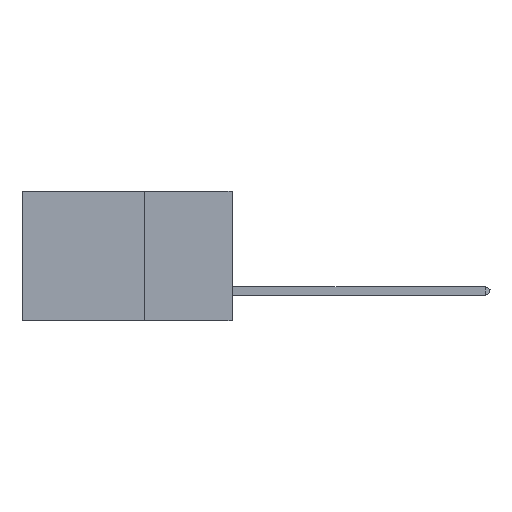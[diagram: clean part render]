
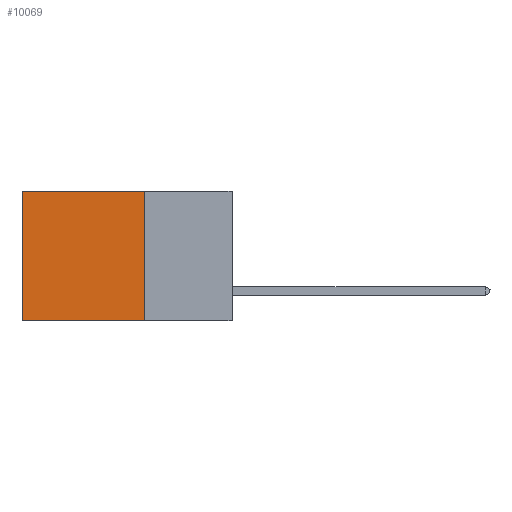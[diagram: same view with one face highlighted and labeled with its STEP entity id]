
A CAD part, left-side view. The second image highlights one B-rep face of the part: STEP entity #10069.
In plain terms, the highlighted planar face has unit normal (-1, 0, 0).
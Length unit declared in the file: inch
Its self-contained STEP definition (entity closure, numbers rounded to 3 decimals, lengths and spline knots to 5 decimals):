
#80 = VERTEX_POINT ( 'NONE', #22462 ) ;
#1959 = LINE ( 'NONE', #12753, #18884 ) ;
#3617 = ORIENTED_EDGE ( 'NONE', *, *, #5419, .T. ) ;
#4255 = CARTESIAN_POINT ( 'NONE',  ( 0.2875, 0.6, -0.37 ) ) ;
#4727 = EDGE_CURVE ( 'NONE', #80, #43732, #26885, .T. ) ;
#4766 = LINE ( 'NONE', #8727, #22227 ) ;
#5419 = EDGE_CURVE ( 'NONE', #16452, #80, #1959, .T. ) ;
#5517 = DIRECTION ( 'NONE',  ( 0., 0., -1. ) ) ;
#6976 = VECTOR ( 'NONE', #5517, 39.37008 ) ;
#8727 = CARTESIAN_POINT ( 'NONE',  ( 0.2875, 0.25, -0.37 ) ) ;
#9321 = DIRECTION ( 'NONE',  ( 0., 1., 0. ) ) ;
#9441 = DIRECTION ( 'NONE',  ( 0., 0., -1. ) ) ;
#10053 = PLANE ( 'NONE',  #28474 ) ;
#10069 = ADVANCED_FACE ( 'NONE', ( #41550 ), #10053, .F. ) ;
#10844 = ORIENTED_EDGE ( 'NONE', *, *, #43040, .F. ) ;
#12753 = CARTESIAN_POINT ( 'NONE',  ( 0.2875, 0.25, 0. ) ) ;
#13505 = DIRECTION ( 'NONE',  ( 0., 0., -1. ) ) ;
#13970 = ORIENTED_EDGE ( 'NONE', *, *, #28134, .F. ) ;
#14473 = CARTESIAN_POINT ( 'NONE',  ( 0.2875, 0.25, 0. ) ) ;
#16452 = VERTEX_POINT ( 'NONE', #23344 ) ;
#18884 = VECTOR ( 'NONE', #9321, 39.37008 ) ;
#19973 = CARTESIAN_POINT ( 'NONE',  ( 0.2875, 0.25, -0.37 ) ) ;
#20167 = CARTESIAN_POINT ( 'NONE',  ( 0.2875, 0.6, 0. ) ) ;
#22227 = VECTOR ( 'NONE', #30052, 39.37008 ) ;
#22462 = CARTESIAN_POINT ( 'NONE',  ( 0.2875, 0.6, 0. ) ) ;
#23344 = CARTESIAN_POINT ( 'NONE',  ( 0.2875, 0.25, 0. ) ) ;
#26885 = LINE ( 'NONE', #20167, #45029 ) ;
#27802 = CARTESIAN_POINT ( 'NONE',  ( 0.2875, 0.25, 0. ) ) ;
#28134 = EDGE_CURVE ( 'NONE', #16452, #32586, #46681, .T. ) ;
#28474 = AXIS2_PLACEMENT_3D ( 'NONE', #14473, #35374, #13505 ) ;
#30052 = DIRECTION ( 'NONE',  ( 0., 1., 0. ) ) ;
#32586 = VERTEX_POINT ( 'NONE', #19973 ) ;
#35374 = DIRECTION ( 'NONE',  ( 1., 0., 0. ) ) ;
#37618 = ORIENTED_EDGE ( 'NONE', *, *, #4727, .T. ) ;
#38547 = EDGE_LOOP ( 'NONE', ( #37618, #10844, #13970, #3617 ) ) ;
#41550 = FACE_OUTER_BOUND ( 'NONE', #38547, .T. ) ;
#43040 = EDGE_CURVE ( 'NONE', #32586, #43732, #4766, .T. ) ;
#43732 = VERTEX_POINT ( 'NONE', #4255 ) ;
#45029 = VECTOR ( 'NONE', #9441, 39.37008 ) ;
#46681 = LINE ( 'NONE', #27802, #6976 ) ;
